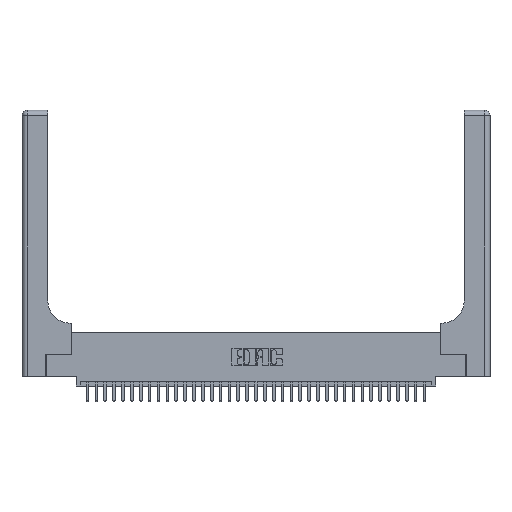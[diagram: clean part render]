
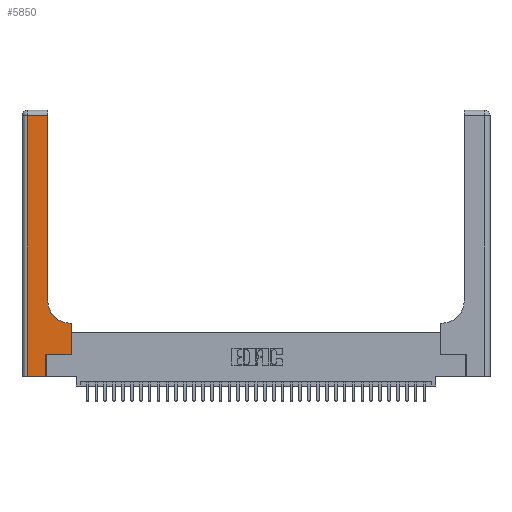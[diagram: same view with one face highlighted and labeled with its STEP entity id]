
A CAD part, top view. The second image highlights one B-rep face of the part: STEP entity #5850.
In plain terms, the highlighted planar face has unit normal (0, 0, 1).
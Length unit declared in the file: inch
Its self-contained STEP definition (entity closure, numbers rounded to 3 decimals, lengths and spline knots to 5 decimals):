
#6 = ORIENTED_EDGE ( 'NONE', *, *, #16352, .T. ) ;
#920 = VERTEX_POINT ( 'NONE', #6164 ) ;
#2045 = ORIENTED_EDGE ( 'NONE', *, *, #32097, .T. ) ;
#2521 = ORIENTED_EDGE ( 'NONE', *, *, #30658, .T. ) ;
#4574 = CARTESIAN_POINT ( 'NONE',  ( 0.5415, 0.6, 0.37 ) ) ;
#4613 = PLANE ( 'NONE',  #17258 ) ;
#4714 = ORIENTED_EDGE ( 'NONE', *, *, #33166, .T. ) ;
#4747 = FACE_OUTER_BOUND ( 'NONE', #11302, .T. ) ;
#4839 = DIRECTION ( 'NONE',  ( 1., 0., 0. ) ) ;
#4874 = VERTEX_POINT ( 'NONE', #9591 ) ;
#5850 = ADVANCED_FACE ( 'NONE', ( #4747 ), #4613, .F. ) ;
#5907 = VECTOR ( 'NONE', #11971, 39.37008 ) ;
#6164 = CARTESIAN_POINT ( 'NONE',  ( 0.06, 0., 0.37 ) ) ;
#6965 = DIRECTION ( 'NONE',  ( 0., 1., 0. ) ) ;
#7354 = VERTEX_POINT ( 'NONE', #29535 ) ;
#7461 = CARTESIAN_POINT ( 'NONE',  ( 0.269, 0.25, 0.37 ) ) ;
#7718 = ORIENTED_EDGE ( 'NONE', *, *, #17088, .T. ) ;
#8046 = VECTOR ( 'NONE', #4839, 39.37008 ) ;
#8108 = VERTEX_POINT ( 'NONE', #7461 ) ;
#8314 = CIRCLE ( 'NONE', #10207, 0.25 ) ;
#8554 = ORIENTED_EDGE ( 'NONE', *, *, #20405, .T. ) ;
#9573 = LINE ( 'NONE', #31580, #16237 ) ;
#9591 = CARTESIAN_POINT ( 'NONE',  ( 0.5585, 0.6, 0.37 ) ) ;
#9930 = DIRECTION ( 'NONE',  ( 1., 0., 0. ) ) ;
#10207 = AXIS2_PLACEMENT_3D ( 'NONE', #18281, #23946, #9930 ) ;
#10617 = CARTESIAN_POINT ( 'NONE',  ( 0.2915, 0.6, 0.37 ) ) ;
#11024 = CARTESIAN_POINT ( 'NONE',  ( 0.5585, 0.25, 0.37 ) ) ;
#11164 = LINE ( 'NONE', #27388, #16031 ) ;
#11302 = EDGE_LOOP ( 'NONE', ( #2521, #6, #4714, #21491, #2045, #31104, #7718, #19589, #8554 ) ) ;
#11406 = VERTEX_POINT ( 'NONE', #17342 ) ;
#11540 = LINE ( 'NONE', #10617, #31317 ) ;
#11693 = VECTOR ( 'NONE', #12036, 39.37008 ) ;
#11971 = DIRECTION ( 'NONE',  ( -1., 0., 0. ) ) ;
#12036 = DIRECTION ( 'NONE',  ( 1., 0., 0. ) ) ;
#12557 = CARTESIAN_POINT ( 'NONE',  ( 0., 3., 0.37 ) ) ;
#13368 = DIRECTION ( 'NONE',  ( 0., -1., 0. ) ) ;
#16031 = VECTOR ( 'NONE', #13368, 39.37008 ) ;
#16074 = LINE ( 'NONE', #24906, #5907 ) ;
#16237 = VECTOR ( 'NONE', #26179, 39.37008 ) ;
#16352 = EDGE_CURVE ( 'NONE', #7354, #19018, #16074, .T. ) ;
#17088 = EDGE_CURVE ( 'NONE', #21419, #4874, #23870, .T. ) ;
#17258 = AXIS2_PLACEMENT_3D ( 'NONE', #12557, #26707, #29672 ) ;
#17342 = CARTESIAN_POINT ( 'NONE',  ( 0.2915, 0.85, 0.37 ) ) ;
#18168 = CARTESIAN_POINT ( 'NONE',  ( 0.269, 0., 0.37 ) ) ;
#18281 = CARTESIAN_POINT ( 'NONE',  ( 0.5415, 0.85, 0.37 ) ) ;
#18728 = DIRECTION ( 'NONE',  ( -1., 0., 0. ) ) ;
#19018 = VERTEX_POINT ( 'NONE', #30030 ) ;
#19589 = ORIENTED_EDGE ( 'NONE', *, *, #28515, .T. ) ;
#20405 = EDGE_CURVE ( 'NONE', #34798, #11406, #8314, .T. ) ;
#21419 = VERTEX_POINT ( 'NONE', #11024 ) ;
#21491 = ORIENTED_EDGE ( 'NONE', *, *, #33821, .T. ) ;
#21729 = DIRECTION ( 'NONE',  ( 0., 1., 0. ) ) ;
#23513 = VECTOR ( 'NONE', #6965, 39.37008 ) ;
#23870 = LINE ( 'NONE', #32687, #30499 ) ;
#23946 = DIRECTION ( 'NONE',  ( 0., 0., -1. ) ) ;
#24051 = LINE ( 'NONE', #35945, #11693 ) ;
#24822 = EDGE_CURVE ( 'NONE', #8108, #21419, #24051, .T. ) ;
#24906 = CARTESIAN_POINT ( 'NONE',  ( 0., 2.94, 0.37 ) ) ;
#25752 = LINE ( 'NONE', #25926, #23513 ) ;
#25926 = CARTESIAN_POINT ( 'NONE',  ( 0.269, 0., 0.37 ) ) ;
#26179 = DIRECTION ( 'NONE',  ( 0., 1., 0. ) ) ;
#26707 = DIRECTION ( 'NONE',  ( 0., 0., -1. ) ) ;
#27388 = CARTESIAN_POINT ( 'NONE',  ( 0.06, 3., 0.37 ) ) ;
#28276 = LINE ( 'NONE', #35991, #8046 ) ;
#28515 = EDGE_CURVE ( 'NONE', #4874, #34798, #11540, .T. ) ;
#29535 = CARTESIAN_POINT ( 'NONE',  ( 0.2915, 2.94, 0.37 ) ) ;
#29672 = DIRECTION ( 'NONE',  ( -1., 0., 0. ) ) ;
#30030 = CARTESIAN_POINT ( 'NONE',  ( 0.06, 2.94, 0.37 ) ) ;
#30499 = VECTOR ( 'NONE', #21729, 39.37008 ) ;
#30658 = EDGE_CURVE ( 'NONE', #11406, #7354, #9573, .T. ) ;
#31104 = ORIENTED_EDGE ( 'NONE', *, *, #24822, .T. ) ;
#31317 = VECTOR ( 'NONE', #18728, 39.37008 ) ;
#31580 = CARTESIAN_POINT ( 'NONE',  ( 0.2915, 3., 0.37 ) ) ;
#32097 = EDGE_CURVE ( 'NONE', #32239, #8108, #25752, .T. ) ;
#32239 = VERTEX_POINT ( 'NONE', #18168 ) ;
#32687 = CARTESIAN_POINT ( 'NONE',  ( 0.5585, 0.25, 0.37 ) ) ;
#33166 = EDGE_CURVE ( 'NONE', #19018, #920, #11164, .T. ) ;
#33821 = EDGE_CURVE ( 'NONE', #920, #32239, #28276, .T. ) ;
#34798 = VERTEX_POINT ( 'NONE', #4574 ) ;
#35945 = CARTESIAN_POINT ( 'NONE',  ( 0.269, 0.25, 0.37 ) ) ;
#35991 = CARTESIAN_POINT ( 'NONE',  ( 0., 0., 0.37 ) ) ;
